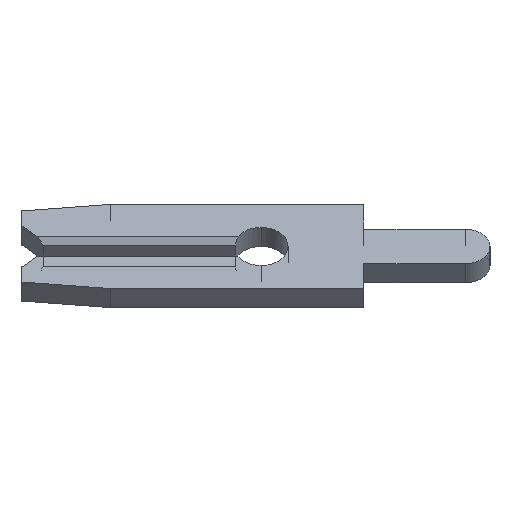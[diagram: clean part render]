
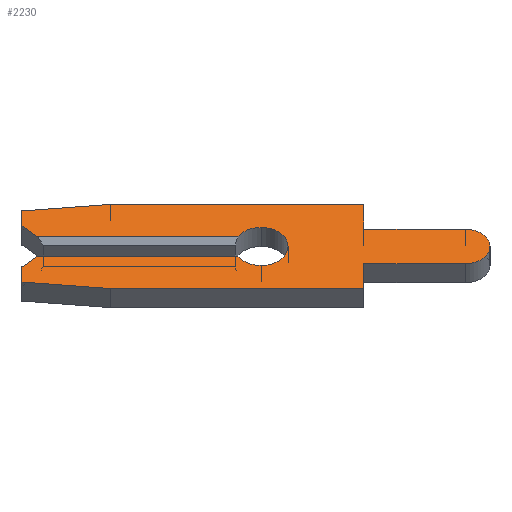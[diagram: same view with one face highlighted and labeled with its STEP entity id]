
A CAD part, left-side view. The second image highlights one B-rep face of the part: STEP entity #2230.
In plain terms, the highlighted face is planar.
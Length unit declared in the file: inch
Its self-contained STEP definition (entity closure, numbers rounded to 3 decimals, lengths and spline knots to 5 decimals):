
#5 = EDGE_CURVE ( 'NONE', #1041, #1541, #1745, .T. ) ;
#32 = LINE ( 'NONE', #193, #2158 ) ;
#48 = VERTEX_POINT ( 'NONE', #93 ) ;
#63 = CARTESIAN_POINT ( 'NONE',  ( -0.013, -0.099, -0.0575 ) ) ;
#68 = VECTOR ( 'NONE', #379, 39.37008 ) ;
#76 = CARTESIAN_POINT ( 'NONE',  ( -0.013, 0.02252, 0.013 ) ) ;
#93 = CARTESIAN_POINT ( 'NONE',  ( -0.013, -0.099, 0.0575 ) ) ;
#97 = CARTESIAN_POINT ( 'NONE',  ( -0.013, 0.2105, 0.0075 ) ) ;
#121 = EDGE_CURVE ( 'NONE', #1541, #336, #1290, .T. ) ;
#124 = EDGE_CURVE ( 'NONE', #336, #1259, #558, .T. ) ;
#132 = DIRECTION ( 'NONE',  ( 0., -1., 0. ) ) ;
#145 = EDGE_CURVE ( 'NONE', #1514, #1041, #1043, .T. ) ;
#187 = CARTESIAN_POINT ( 'NONE',  ( -0.013, 0., -0.013 ) ) ;
#193 = CARTESIAN_POINT ( 'NONE',  ( -0.013, 0.146, -0.0575 ) ) ;
#203 = VECTOR ( 'NONE', #1311, 39.37008 ) ;
#216 = CARTESIAN_POINT ( 'NONE',  ( -0.013, 0.231, 0.028 ) ) ;
#228 = ORIENTED_EDGE ( 'NONE', *, *, #1357, .F. ) ;
#230 = CARTESIAN_POINT ( 'NONE',  ( -0.013, 0.02252, -0.013 ) ) ;
#239 = CARTESIAN_POINT ( 'NONE',  ( -0.013, -0.099, -0.0235 ) ) ;
#241 = EDGE_CURVE ( 'NONE', #1828, #604, #1718, .T. ) ;
#266 = ORIENTED_EDGE ( 'NONE', *, *, #1896, .F. ) ;
#283 = CARTESIAN_POINT ( 'NONE',  ( -0.013, -0.099, 0.0575 ) ) ;
#294 = VERTEX_POINT ( 'NONE', #579 ) ;
#295 = ORIENTED_EDGE ( 'NONE', *, *, #145, .F. ) ;
#313 = VERTEX_POINT ( 'NONE', #921 ) ;
#324 = CARTESIAN_POINT ( 'NONE',  ( -0.013, 0.231, 0.04857 ) ) ;
#336 = VERTEX_POINT ( 'NONE', #1124 ) ;
#349 = DIRECTION ( 'NONE',  ( 0., 0., 1. ) ) ;
#358 = AXIS2_PLACEMENT_3D ( 'NONE', #1581, #1589, #710 ) ;
#367 = ORIENTED_EDGE ( 'NONE', *, *, #518, .F. ) ;
#379 = DIRECTION ( 'NONE',  ( 0., 1., 0. ) ) ;
#402 = VECTOR ( 'NONE', #1465, 39.37008 ) ;
#408 = VECTOR ( 'NONE', #1530, 39.37008 ) ;
#414 = CARTESIAN_POINT ( 'NONE',  ( -0.013, -0.099, 0.0235 ) ) ;
#476 = VERTEX_POINT ( 'NONE', #414 ) ;
#518 = EDGE_CURVE ( 'NONE', #1961, #294, #874, .T. ) ;
#542 = CARTESIAN_POINT ( 'NONE',  ( -0.013, 0.146, -0.0575 ) ) ;
#546 = EDGE_CURVE ( 'NONE', #1782, #2229, #2219, .T. ) ;
#558 = CIRCLE ( 'NONE', #1854, 0.026 ) ;
#561 = CARTESIAN_POINT ( 'NONE',  ( -0.013, -0.1975, -0.0235 ) ) ;
#564 = CARTESIAN_POINT ( 'NONE',  ( -0.013, 0.231, -0.028 ) ) ;
#579 = CARTESIAN_POINT ( 'NONE',  ( -0.013, -0.099, -0.0235 ) ) ;
#598 = CARTESIAN_POINT ( 'NONE',  ( -0.013, 0.216, 0.013 ) ) ;
#604 = VERTEX_POINT ( 'NONE', #763 ) ;
#682 = VERTEX_POINT ( 'NONE', #598 ) ;
#689 = VERTEX_POINT ( 'NONE', #542 ) ;
#710 = DIRECTION ( 'NONE',  ( 0., 0., -1. ) ) ;
#712 = AXIS2_PLACEMENT_3D ( 'NONE', #1596, #1239, #728 ) ;
#728 = DIRECTION ( 'NONE',  ( 0., 0., -1. ) ) ;
#730 = DIRECTION ( 'NONE',  ( 0., 1., 0. ) ) ;
#747 = ORIENTED_EDGE ( 'NONE', *, *, #5, .F. ) ;
#763 = CARTESIAN_POINT ( 'NONE',  ( -0.013, 0.146, 0.0575 ) ) ;
#764 = VECTOR ( 'NONE', #1375, 39.37008 ) ;
#781 = DIRECTION ( 'NONE',  ( 0., 0., -1. ) ) ;
#862 = ORIENTED_EDGE ( 'NONE', *, *, #1407, .F. ) ;
#874 = LINE ( 'NONE', #239, #68 ) ;
#921 = CARTESIAN_POINT ( 'NONE',  ( -0.013, -0.099, -0.0575 ) ) ;
#932 = VERTEX_POINT ( 'NONE', #216 ) ;
#939 = VECTOR ( 'NONE', #132, 39.37008 ) ;
#992 = ORIENTED_EDGE ( 'NONE', *, *, #1242, .F. ) ;
#1011 = FACE_OUTER_BOUND ( 'NONE', #1883, .T. ) ;
#1021 = CARTESIAN_POINT ( 'NONE',  ( -0.013, 0.2105, -0.0075 ) ) ;
#1041 = VERTEX_POINT ( 'NONE', #230 ) ;
#1043 = LINE ( 'NONE', #187, #2027 ) ;
#1059 = VECTOR ( 'NONE', #349, 39.37008 ) ;
#1080 = DIRECTION ( 'NONE',  ( 0., 0., -1. ) ) ;
#1081 = ORIENTED_EDGE ( 'NONE', *, *, #2177, .F. ) ;
#1085 = DIRECTION ( 'NONE',  ( -1., 0., 0. ) ) ;
#1103 = CARTESIAN_POINT ( 'NONE',  ( -0.013, 0., 0. ) ) ;
#1124 = CARTESIAN_POINT ( 'NONE',  ( -0.013, 0., 0.026 ) ) ;
#1187 = VECTOR ( 'NONE', #1356, 39.37008 ) ;
#1193 = ORIENTED_EDGE ( 'NONE', *, *, #1355, .F. ) ;
#1198 = EDGE_CURVE ( 'NONE', #476, #1754, #1265, .T. ) ;
#1231 = ORIENTED_EDGE ( 'NONE', *, *, #546, .F. ) ;
#1238 = LINE ( 'NONE', #1694, #1187 ) ;
#1239 = DIRECTION ( 'NONE',  ( -1., 0., 0. ) ) ;
#1242 = EDGE_CURVE ( 'NONE', #294, #313, #1867, .T. ) ;
#1244 = DIRECTION ( 'NONE',  ( 0., 0., -1. ) ) ;
#1249 = DIRECTION ( 'NONE',  ( 0., -1., 0. ) ) ;
#1259 = VERTEX_POINT ( 'NONE', #76 ) ;
#1265 = LINE ( 'NONE', #1810, #203 ) ;
#1268 = PLANE ( 'NONE',  #1615 ) ;
#1290 = CIRCLE ( 'NONE', #358, 0.026 ) ;
#1296 = VECTOR ( 'NONE', #781, 39.37008 ) ;
#1311 = DIRECTION ( 'NONE',  ( 0., -1., 0. ) ) ;
#1355 = EDGE_CURVE ( 'NONE', #682, #932, #1511, .T. ) ;
#1356 = DIRECTION ( 'NONE',  ( 0., 0.995, 0.105 ) ) ;
#1357 = EDGE_CURVE ( 'NONE', #48, #476, #1406, .T. ) ;
#1368 = ORIENTED_EDGE ( 'NONE', *, *, #121, .F. ) ;
#1370 = ORIENTED_EDGE ( 'NONE', *, *, #2176, .F. ) ;
#1375 = DIRECTION ( 'NONE',  ( 0., -0.707, 0.707 ) ) ;
#1376 = CIRCLE ( 'NONE', #1861, 0.0235 ) ;
#1406 = LINE ( 'NONE', #283, #2195 ) ;
#1407 = EDGE_CURVE ( 'NONE', #689, #1782, #1238, .T. ) ;
#1430 = EDGE_CURVE ( 'NONE', #1754, #1961, #1376, .T. ) ;
#1442 = DIRECTION ( 'NONE',  ( 0., -1., 0. ) ) ;
#1465 = DIRECTION ( 'NONE',  ( 0., 0., 1. ) ) ;
#1475 = VECTOR ( 'NONE', #1249, 39.37008 ) ;
#1505 = EDGE_CURVE ( 'NONE', #2229, #1514, #1611, .T. ) ;
#1507 = EDGE_CURVE ( 'NONE', #682, #1259, #2169, .T. ) ;
#1511 = LINE ( 'NONE', #97, #408 ) ;
#1514 = VERTEX_POINT ( 'NONE', #2054 ) ;
#1528 = DIRECTION ( 'NONE',  ( 1., 0., 0. ) ) ;
#1530 = DIRECTION ( 'NONE',  ( 0., 0.707, 0.707 ) ) ;
#1541 = VERTEX_POINT ( 'NONE', #1717 ) ;
#1559 = DIRECTION ( 'NONE',  ( 0., 0., -1. ) ) ;
#1581 = CARTESIAN_POINT ( 'NONE',  ( -0.013, 0., 0. ) ) ;
#1584 = DIRECTION ( 'NONE',  ( 1., 0., 0. ) ) ;
#1589 = DIRECTION ( 'NONE',  ( -1., 0., 0. ) ) ;
#1594 = ORIENTED_EDGE ( 'NONE', *, *, #241, .F. ) ;
#1596 = CARTESIAN_POINT ( 'NONE',  ( -0.013, 0., 0. ) ) ;
#1611 = LINE ( 'NONE', #1021, #764 ) ;
#1615 = AXIS2_PLACEMENT_3D ( 'NONE', #1103, #1584, #1080 ) ;
#1636 = ORIENTED_EDGE ( 'NONE', *, *, #1505, .F. ) ;
#1694 = CARTESIAN_POINT ( 'NONE',  ( -0.013, 0.231, -0.04857 ) ) ;
#1712 = ORIENTED_EDGE ( 'NONE', *, *, #124, .F. ) ;
#1717 = CARTESIAN_POINT ( 'NONE',  ( -0.013, 0., -0.026 ) ) ;
#1718 = LINE ( 'NONE', #1980, #1888 ) ;
#1745 = CIRCLE ( 'NONE', #712, 0.026 ) ;
#1749 = CARTESIAN_POINT ( 'NONE',  ( -0.013, 0.231, 0.028 ) ) ;
#1754 = VERTEX_POINT ( 'NONE', #2091 ) ;
#1782 = VERTEX_POINT ( 'NONE', #1938 ) ;
#1810 = CARTESIAN_POINT ( 'NONE',  ( -0.013, -0.099, 0.0235 ) ) ;
#1815 = DIRECTION ( 'NONE',  ( 0., -0.995, 0.105 ) ) ;
#1828 = VERTEX_POINT ( 'NONE', #324 ) ;
#1843 = ORIENTED_EDGE ( 'NONE', *, *, #1430, .F. ) ;
#1854 = AXIS2_PLACEMENT_3D ( 'NONE', #1955, #1085, #1244 ) ;
#1860 = ORIENTED_EDGE ( 'NONE', *, *, #1507, .T. ) ;
#1861 = AXIS2_PLACEMENT_3D ( 'NONE', #2248, #1528, #2234 ) ;
#1867 = LINE ( 'NONE', #63, #1296 ) ;
#1883 = EDGE_LOOP ( 'NONE', ( #1860, #1712, #1368, #747, #295, #1636, #1231, #862, #1081, #992, #367, #1843, #2034, #228, #1370, #1594, #266, #1193 ) ) ;
#1888 = VECTOR ( 'NONE', #1815, 39.37008 ) ;
#1896 = EDGE_CURVE ( 'NONE', #932, #1828, #2214, .T. ) ;
#1938 = CARTESIAN_POINT ( 'NONE',  ( -0.013, 0.231, -0.04857 ) ) ;
#1947 = CARTESIAN_POINT ( 'NONE',  ( -0.013, 0.146, 0.0575 ) ) ;
#1955 = CARTESIAN_POINT ( 'NONE',  ( -0.013, 0., 0. ) ) ;
#1961 = VERTEX_POINT ( 'NONE', #561 ) ;
#1980 = CARTESIAN_POINT ( 'NONE',  ( -0.013, 0.231, 0.04857 ) ) ;
#2027 = VECTOR ( 'NONE', #1442, 39.37008 ) ;
#2034 = ORIENTED_EDGE ( 'NONE', *, *, #1198, .F. ) ;
#2054 = CARTESIAN_POINT ( 'NONE',  ( -0.013, 0.216, -0.013 ) ) ;
#2073 = LINE ( 'NONE', #1947, #1475 ) ;
#2091 = CARTESIAN_POINT ( 'NONE',  ( -0.013, -0.1975, 0.0235 ) ) ;
#2125 = CARTESIAN_POINT ( 'NONE',  ( -0.013, 0.231, -0.028 ) ) ;
#2158 = VECTOR ( 'NONE', #730, 39.37008 ) ;
#2169 = LINE ( 'NONE', #2223, #939 ) ;
#2176 = EDGE_CURVE ( 'NONE', #604, #48, #2073, .T. ) ;
#2177 = EDGE_CURVE ( 'NONE', #313, #689, #32, .T. ) ;
#2195 = VECTOR ( 'NONE', #1559, 39.37008 ) ;
#2214 = LINE ( 'NONE', #1749, #1059 ) ;
#2219 = LINE ( 'NONE', #564, #402 ) ;
#2223 = CARTESIAN_POINT ( 'NONE',  ( -0.013, 0.231, 0.013 ) ) ;
#2229 = VERTEX_POINT ( 'NONE', #2125 ) ;
#2230 = ADVANCED_FACE ( 'NONE', ( #1011 ), #1268, .F. ) ;
#2234 = DIRECTION ( 'NONE',  ( 0., 0., 1. ) ) ;
#2248 = CARTESIAN_POINT ( 'NONE',  ( -0.013, -0.1975, 0. ) ) ;
